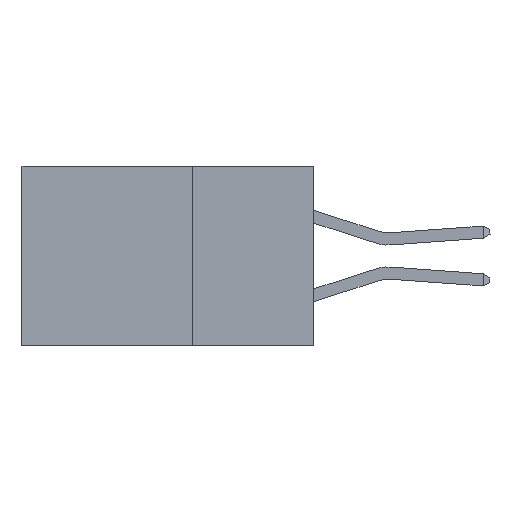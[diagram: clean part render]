
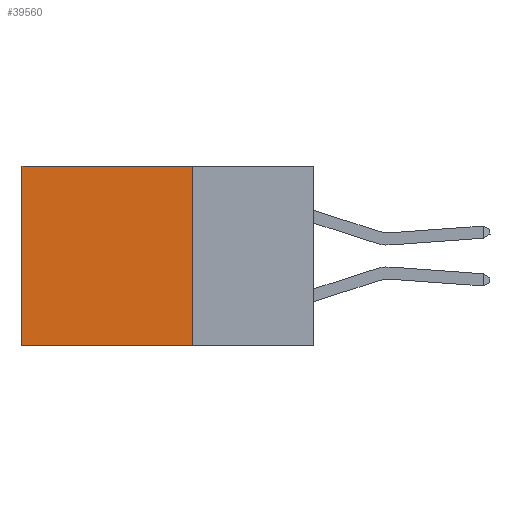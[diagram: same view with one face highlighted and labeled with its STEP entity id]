
A CAD part, left-side view. The second image highlights one B-rep face of the part: STEP entity #39560.
In plain terms, the highlighted planar face has unit normal (-1, 0, 0).
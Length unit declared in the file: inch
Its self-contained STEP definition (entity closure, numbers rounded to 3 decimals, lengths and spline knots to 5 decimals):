
#406 = CARTESIAN_POINT ( 'NONE',  ( 0.2875, 0.6, 0. ) ) ;
#1427 = CARTESIAN_POINT ( 'NONE',  ( 0.2875, 0.6, -0.37 ) ) ;
#2316 = CARTESIAN_POINT ( 'NONE',  ( 0.2875, 0.25, 0. ) ) ;
#2523 = ORIENTED_EDGE ( 'NONE', *, *, #25254, .T. ) ;
#3367 = AXIS2_PLACEMENT_3D ( 'NONE', #23384, #26525, #20173 ) ;
#4410 = PLANE ( 'NONE',  #3367 ) ;
#6316 = LINE ( 'NONE', #26124, #7331 ) ;
#6787 = CARTESIAN_POINT ( 'NONE',  ( 0.2875, 0.6, 0. ) ) ;
#7331 = VECTOR ( 'NONE', #10674, 39.37008 ) ;
#7771 = CARTESIAN_POINT ( 'NONE',  ( 0.2875, 0.25, -0.37 ) ) ;
#9993 = VECTOR ( 'NONE', #34306, 39.37008 ) ;
#10674 = DIRECTION ( 'NONE',  ( 0., 0., -1. ) ) ;
#14001 = VERTEX_POINT ( 'NONE', #21795 ) ;
#16867 = ORIENTED_EDGE ( 'NONE', *, *, #22754, .F. ) ;
#17596 = VERTEX_POINT ( 'NONE', #406 ) ;
#17800 = VECTOR ( 'NONE', #18277, 39.37008 ) ;
#18277 = DIRECTION ( 'NONE',  ( 0., 1., 0. ) ) ;
#19548 = EDGE_LOOP ( 'NONE', ( #33498, #31525, #16867, #2523 ) ) ;
#20173 = DIRECTION ( 'NONE',  ( 0., 0., -1. ) ) ;
#21795 = CARTESIAN_POINT ( 'NONE',  ( 0.2875, 0.25, 0. ) ) ;
#22754 = EDGE_CURVE ( 'NONE', #14001, #35314, #6316, .T. ) ;
#23384 = CARTESIAN_POINT ( 'NONE',  ( 0.2875, 0.25, 0. ) ) ;
#23460 = VERTEX_POINT ( 'NONE', #1427 ) ;
#24952 = CARTESIAN_POINT ( 'NONE',  ( 0.2875, 0.25, -0.37 ) ) ;
#25254 = EDGE_CURVE ( 'NONE', #14001, #17596, #29943, .T. ) ;
#26124 = CARTESIAN_POINT ( 'NONE',  ( 0.2875, 0.25, 0. ) ) ;
#26525 = DIRECTION ( 'NONE',  ( 1., 0., 0. ) ) ;
#26872 = VECTOR ( 'NONE', #37811, 39.37008 ) ;
#26934 = EDGE_CURVE ( 'NONE', #17596, #23460, #38479, .T. ) ;
#29943 = LINE ( 'NONE', #2316, #17800 ) ;
#31525 = ORIENTED_EDGE ( 'NONE', *, *, #37644, .F. ) ;
#33498 = ORIENTED_EDGE ( 'NONE', *, *, #26934, .T. ) ;
#34306 = DIRECTION ( 'NONE',  ( 0., 1., 0. ) ) ;
#35314 = VERTEX_POINT ( 'NONE', #7771 ) ;
#37644 = EDGE_CURVE ( 'NONE', #35314, #23460, #38614, .T. ) ;
#37811 = DIRECTION ( 'NONE',  ( 0., 0., -1. ) ) ;
#38479 = LINE ( 'NONE', #6787, #26872 ) ;
#38614 = LINE ( 'NONE', #24952, #9993 ) ;
#39560 = ADVANCED_FACE ( 'NONE', ( #40096 ), #4410, .F. ) ;
#40096 = FACE_OUTER_BOUND ( 'NONE', #19548, .T. ) ;
